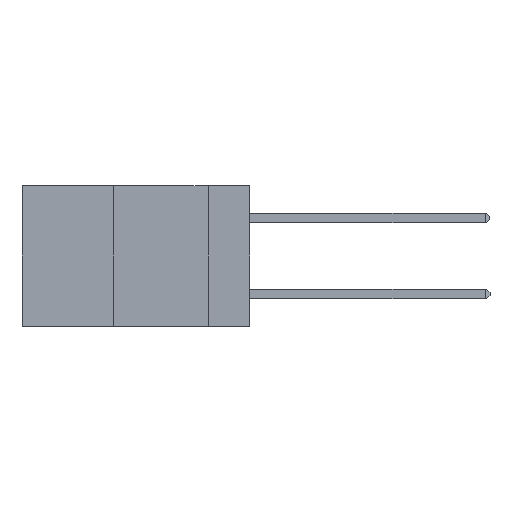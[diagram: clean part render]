
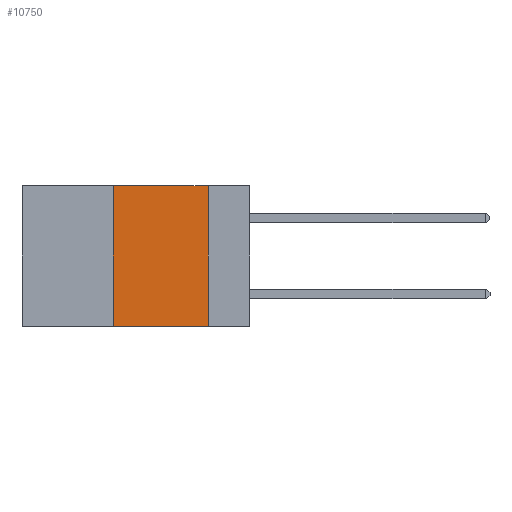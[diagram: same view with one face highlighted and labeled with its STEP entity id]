
A CAD part, left-side view. The second image highlights one B-rep face of the part: STEP entity #10750.
In plain terms, the highlighted planar face has unit normal (-1, 0, 0).
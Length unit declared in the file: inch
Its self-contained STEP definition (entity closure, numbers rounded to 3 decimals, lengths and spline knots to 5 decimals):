
#1125 = VERTEX_POINT ( 'NONE', #2641 ) ;
#2641 = CARTESIAN_POINT ( 'NONE',  ( 0., 0.36, -0.37 ) ) ;
#3115 = VECTOR ( 'NONE', #5042, 39.37008 ) ;
#3215 = CARTESIAN_POINT ( 'NONE',  ( 0., 0.36, 0. ) ) ;
#3919 = PLANE ( 'NONE',  #15852 ) ;
#4100 = EDGE_CURVE ( 'NONE', #12514, #15903, #8881, .T. ) ;
#5042 = DIRECTION ( 'NONE',  ( 0., -1., 0. ) ) ;
#6833 = CARTESIAN_POINT ( 'NONE',  ( 0., 0.11, 0. ) ) ;
#7153 = DIRECTION ( 'NONE',  ( 1., 0., 0. ) ) ;
#7537 = CARTESIAN_POINT ( 'NONE',  ( 0., 0.11, -0.37 ) ) ;
#8401 = VECTOR ( 'NONE', #11727, 39.37008 ) ;
#8493 = EDGE_LOOP ( 'NONE', ( #13081, #9371, #14614, #20492 ) ) ;
#8635 = CARTESIAN_POINT ( 'NONE',  ( 0., 0.11, 0. ) ) ;
#8652 = CARTESIAN_POINT ( 'NONE',  ( 0., 0.6, -0.37 ) ) ;
#8881 = LINE ( 'NONE', #8635, #8401 ) ;
#9371 = ORIENTED_EDGE ( 'NONE', *, *, #20643, .F. ) ;
#10458 = EDGE_CURVE ( 'NONE', #1125, #19728, #16601, .T. ) ;
#10580 = FACE_OUTER_BOUND ( 'NONE', #8493, .T. ) ;
#10673 = LINE ( 'NONE', #8652, #14436 ) ;
#10750 = ADVANCED_FACE ( 'NONE', ( #10580 ), #3919, .F. ) ;
#11158 = DIRECTION ( 'NONE',  ( 0., 0., 1. ) ) ;
#11346 = CARTESIAN_POINT ( 'NONE',  ( 0., 0.6, 0. ) ) ;
#11727 = DIRECTION ( 'NONE',  ( 0., 0., -1. ) ) ;
#12317 = VECTOR ( 'NONE', #11158, 39.37008 ) ;
#12514 = VERTEX_POINT ( 'NONE', #6833 ) ;
#13081 = ORIENTED_EDGE ( 'NONE', *, *, #4100, .F. ) ;
#13621 = CARTESIAN_POINT ( 'NONE',  ( 0., 0.36, 0. ) ) ;
#14436 = VECTOR ( 'NONE', #18314, 39.37008 ) ;
#14614 = ORIENTED_EDGE ( 'NONE', *, *, #10458, .F. ) ;
#15163 = EDGE_CURVE ( 'NONE', #1125, #15903, #10673, .T. ) ;
#15852 = AXIS2_PLACEMENT_3D ( 'NONE', #16670, #7153, #18267 ) ;
#15903 = VERTEX_POINT ( 'NONE', #7537 ) ;
#16601 = LINE ( 'NONE', #3215, #12317 ) ;
#16670 = CARTESIAN_POINT ( 'NONE',  ( 0., 0.6, 0. ) ) ;
#18267 = DIRECTION ( 'NONE',  ( 0., 0., -1. ) ) ;
#18314 = DIRECTION ( 'NONE',  ( 0., -1., 0. ) ) ;
#19728 = VERTEX_POINT ( 'NONE', #13621 ) ;
#20012 = LINE ( 'NONE', #11346, #3115 ) ;
#20492 = ORIENTED_EDGE ( 'NONE', *, *, #15163, .T. ) ;
#20643 = EDGE_CURVE ( 'NONE', #19728, #12514, #20012, .T. ) ;
